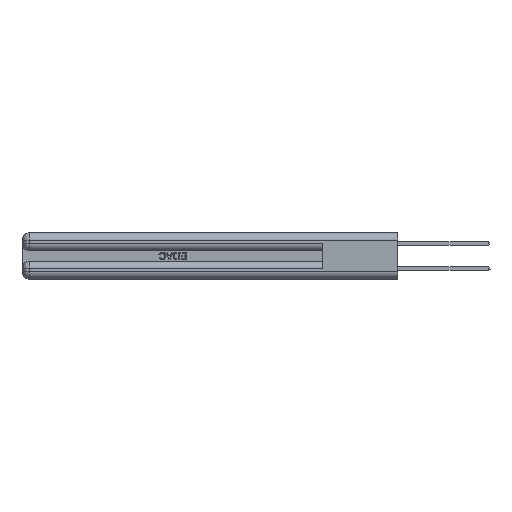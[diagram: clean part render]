
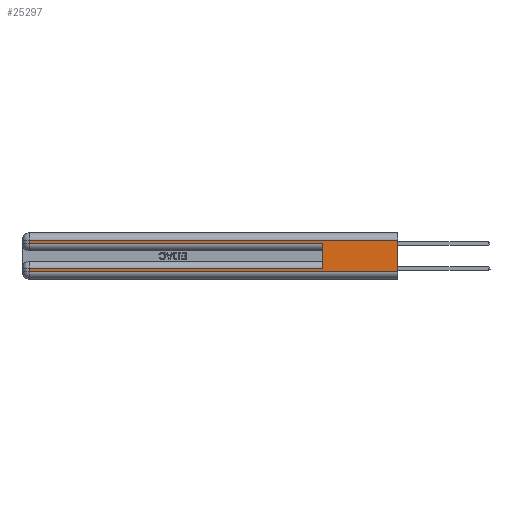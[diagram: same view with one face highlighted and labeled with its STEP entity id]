
A CAD part, left-side view. The second image highlights one B-rep face of the part: STEP entity #25297.
In plain terms, the highlighted planar face has unit normal (-1, 0, 0).
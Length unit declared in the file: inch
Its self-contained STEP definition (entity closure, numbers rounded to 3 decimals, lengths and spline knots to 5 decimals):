
#490 = CARTESIAN_POINT ( 'NONE',  ( 0., 0., 0.285 ) ) ;
#1518 = VECTOR ( 'NONE', #46897, 39.37008 ) ;
#1694 = CARTESIAN_POINT ( 'NONE',  ( 0., 2.94, 0.085 ) ) ;
#3421 = EDGE_CURVE ( 'NONE', #31013, #31870, #3902, .T. ) ;
#3492 = VERTEX_POINT ( 'NONE', #18737 ) ;
#3648 = CARTESIAN_POINT ( 'NONE',  ( 0., 0.6, 0.085 ) ) ;
#3902 = LINE ( 'NONE', #44946, #41019 ) ;
#4339 = VECTOR ( 'NONE', #24439, 39.37008 ) ;
#4689 = DIRECTION ( 'NONE',  ( 0., 0., -1. ) ) ;
#4853 = AXIS2_PLACEMENT_3D ( 'NONE', #11367, #7877, #4689 ) ;
#4960 = EDGE_CURVE ( 'NONE', #31870, #19945, #7276, .T. ) ;
#5657 = ORIENTED_EDGE ( 'NONE', *, *, #45117, .T. ) ;
#7137 = EDGE_CURVE ( 'NONE', #17864, #19945, #33361, .T. ) ;
#7276 = LINE ( 'NONE', #24736, #1518 ) ;
#7877 = DIRECTION ( 'NONE',  ( 1., 0., 0. ) ) ;
#8958 = DIRECTION ( 'NONE',  ( 0., 1., 0. ) ) ;
#11367 = CARTESIAN_POINT ( 'NONE',  ( 0., 0., 0.37 ) ) ;
#13417 = CARTESIAN_POINT ( 'NONE',  ( 0., 0., 0.31 ) ) ;
#14081 = LINE ( 'NONE', #42104, #4339 ) ;
#15395 = DIRECTION ( 'NONE',  ( 0., 0., -1. ) ) ;
#15400 = CARTESIAN_POINT ( 'NONE',  ( 0., 2.94, 0.06 ) ) ;
#15600 = VECTOR ( 'NONE', #28637, 39.37008 ) ;
#17357 = CARTESIAN_POINT ( 'NONE',  ( 0., 0.6, 0.145 ) ) ;
#17864 = VERTEX_POINT ( 'NONE', #35257 ) ;
#18379 = LINE ( 'NONE', #490, #31593 ) ;
#18737 = CARTESIAN_POINT ( 'NONE',  ( 0., 0.6, 0.285 ) ) ;
#19028 = FACE_OUTER_BOUND ( 'NONE', #41991, .T. ) ;
#19945 = VERTEX_POINT ( 'NONE', #44239 ) ;
#21191 = VERTEX_POINT ( 'NONE', #33316 ) ;
#21570 = LINE ( 'NONE', #17357, #34139 ) ;
#22258 = EDGE_CURVE ( 'NONE', #22575, #3492, #21570, .T. ) ;
#22575 = VERTEX_POINT ( 'NONE', #3648 ) ;
#23010 = EDGE_CURVE ( 'NONE', #40064, #21191, #14081, .T. ) ;
#24201 = EDGE_CURVE ( 'NONE', #22575, #31013, #29952, .T. ) ;
#24439 = DIRECTION ( 'NONE',  ( 0., 0., -1. ) ) ;
#24656 = DIRECTION ( 'NONE',  ( 0., 1., 0. ) ) ;
#24736 = CARTESIAN_POINT ( 'NONE',  ( 0., 0., 0.06 ) ) ;
#25297 = ADVANCED_FACE ( 'NONE', ( #19028 ), #44763, .F. ) ;
#26706 = VECTOR ( 'NONE', #24656, 39.37008 ) ;
#26919 = ORIENTED_EDGE ( 'NONE', *, *, #24201, .T. ) ;
#28483 = CARTESIAN_POINT ( 'NONE',  ( 0., 0., 0.37 ) ) ;
#28560 = ORIENTED_EDGE ( 'NONE', *, *, #22258, .F. ) ;
#28637 = DIRECTION ( 'NONE',  ( 0., 0., -1. ) ) ;
#28705 = DIRECTION ( 'NONE',  ( 0., 0., 1. ) ) ;
#28711 = CARTESIAN_POINT ( 'NONE',  ( 0., 2.94, 0.31 ) ) ;
#29548 = ORIENTED_EDGE ( 'NONE', *, *, #3421, .T. ) ;
#29952 = LINE ( 'NONE', #34360, #43621 ) ;
#31013 = VERTEX_POINT ( 'NONE', #1694 ) ;
#31593 = VECTOR ( 'NONE', #44588, 39.37008 ) ;
#31870 = VERTEX_POINT ( 'NONE', #15400 ) ;
#32296 = ORIENTED_EDGE ( 'NONE', *, *, #7137, .F. ) ;
#33316 = CARTESIAN_POINT ( 'NONE',  ( 0., 2.94, 0.285 ) ) ;
#33361 = LINE ( 'NONE', #28483, #15600 ) ;
#34139 = VECTOR ( 'NONE', #28705, 39.37008 ) ;
#34360 = CARTESIAN_POINT ( 'NONE',  ( 0., 0., 0.085 ) ) ;
#35257 = CARTESIAN_POINT ( 'NONE',  ( 0., 0., 0.31 ) ) ;
#36885 = ORIENTED_EDGE ( 'NONE', *, *, #4960, .T. ) ;
#40064 = VERTEX_POINT ( 'NONE', #28711 ) ;
#40321 = EDGE_CURVE ( 'NONE', #21191, #3492, #18379, .T. ) ;
#41019 = VECTOR ( 'NONE', #15395, 39.37008 ) ;
#41991 = EDGE_LOOP ( 'NONE', ( #32296, #5657, #42598, #44208, #28560, #26919, #29548, #36885 ) ) ;
#42104 = CARTESIAN_POINT ( 'NONE',  ( 0., 2.94, 0.37 ) ) ;
#42129 = LINE ( 'NONE', #13417, #26706 ) ;
#42598 = ORIENTED_EDGE ( 'NONE', *, *, #23010, .T. ) ;
#43621 = VECTOR ( 'NONE', #8958, 39.37008 ) ;
#44208 = ORIENTED_EDGE ( 'NONE', *, *, #40321, .T. ) ;
#44239 = CARTESIAN_POINT ( 'NONE',  ( 0., 0., 0.06 ) ) ;
#44588 = DIRECTION ( 'NONE',  ( 0., -1., 0. ) ) ;
#44763 = PLANE ( 'NONE',  #4853 ) ;
#44946 = CARTESIAN_POINT ( 'NONE',  ( 0., 2.94, 0.37 ) ) ;
#45117 = EDGE_CURVE ( 'NONE', #17864, #40064, #42129, .T. ) ;
#46897 = DIRECTION ( 'NONE',  ( 0., -1., 0. ) ) ;
